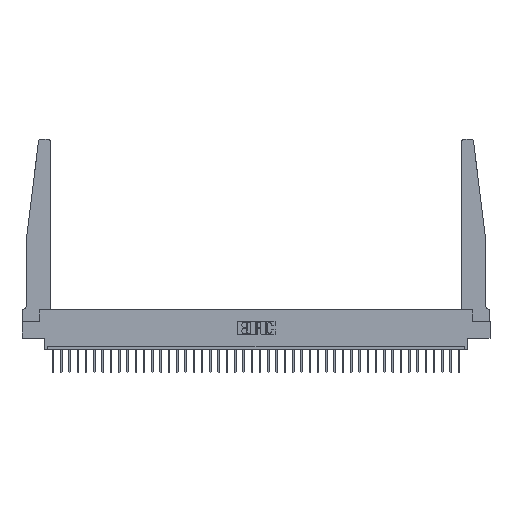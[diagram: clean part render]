
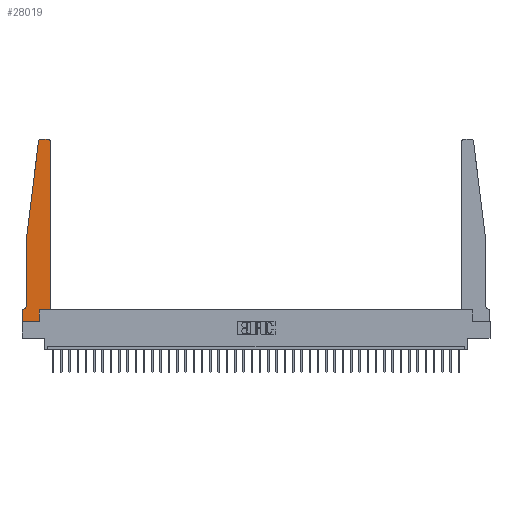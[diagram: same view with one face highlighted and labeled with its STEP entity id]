
A CAD part, top view. The second image highlights one B-rep face of the part: STEP entity #28019.
In plain terms, the highlighted planar face has unit normal (0, 0, 1).
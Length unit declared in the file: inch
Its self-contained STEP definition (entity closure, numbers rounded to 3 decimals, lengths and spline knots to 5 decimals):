
#20 = CARTESIAN_POINT ( 'NONE',  ( 0.015, 0.2375, 0.37 ) ) ;
#563 = EDGE_CURVE ( 'NONE', #23063, #26368, #12569, .T. ) ;
#759 = CARTESIAN_POINT ( 'NONE',  ( 0.425, 0.18, 0.37 ) ) ;
#1128 = CARTESIAN_POINT ( 'NONE',  ( 0.425, 0.18, 0.37 ) ) ;
#1608 = CARTESIAN_POINT ( 'NONE',  ( 0.27653, 2.75, 0.37 ) ) ;
#1908 = LINE ( 'NONE', #4752, #3037 ) ;
#2266 = EDGE_CURVE ( 'NONE', #28816, #15659, #31249, .T. ) ;
#2696 = DIRECTION ( 'NONE',  ( 0., 0., -1. ) ) ;
#2942 = ORIENTED_EDGE ( 'NONE', *, *, #29391, .T. ) ;
#2980 = EDGE_CURVE ( 'NONE', #21040, #24756, #8687, .T. ) ;
#3037 = VECTOR ( 'NONE', #24036, 39.37008 ) ;
#3218 = VERTEX_POINT ( 'NONE', #23481 ) ;
#4462 = LINE ( 'NONE', #7508, #11585 ) ;
#4684 = VERTEX_POINT ( 'NONE', #16471 ) ;
#4752 = CARTESIAN_POINT ( 'NONE',  ( 0.25, 2.75, 0.37 ) ) ;
#4827 = VECTOR ( 'NONE', #22648, 39.37008 ) ;
#4840 = ORIENTED_EDGE ( 'NONE', *, *, #563, .T. ) ;
#4937 = DIRECTION ( 'NONE',  ( 1., 0., 0. ) ) ;
#5009 = ORIENTED_EDGE ( 'NONE', *, *, #22281, .T. ) ;
#5348 = VECTOR ( 'NONE', #34368, 39.37008 ) ;
#5630 = DIRECTION ( 'NONE',  ( 0., 0., 1. ) ) ;
#5675 = EDGE_CURVE ( 'NONE', #25579, #21040, #12344, .T. ) ;
#5929 = ORIENTED_EDGE ( 'NONE', *, *, #35224, .T. ) ;
#6395 = VECTOR ( 'NONE', #9640, 39.37008 ) ;
#6528 = ORIENTED_EDGE ( 'NONE', *, *, #2980, .T. ) ;
#6663 = CARTESIAN_POINT ( 'NONE',  ( 0.425, 0.18, 0.37 ) ) ;
#6870 = LINE ( 'NONE', #7040, #10419 ) ;
#6914 = VECTOR ( 'NONE', #19304, 39.37008 ) ;
#7040 = CARTESIAN_POINT ( 'NONE',  ( 0., 0., 0.37 ) ) ;
#7508 = CARTESIAN_POINT ( 'NONE',  ( 0., 0., 0.37 ) ) ;
#8687 = CIRCLE ( 'NONE', #12109, 0.03 ) ;
#9262 = CARTESIAN_POINT ( 'NONE',  ( 0.065, 1.25, 0.37 ) ) ;
#9301 = AXIS2_PLACEMENT_3D ( 'NONE', #21191, #19019, #4937 ) ;
#9640 = DIRECTION ( 'NONE',  ( -1., 0., 0. ) ) ;
#9796 = VERTEX_POINT ( 'NONE', #22073 ) ;
#10419 = VECTOR ( 'NONE', #31155, 39.37008 ) ;
#11344 = CARTESIAN_POINT ( 'NONE',  ( 0.395, 2.72, 0.37 ) ) ;
#11585 = VECTOR ( 'NONE', #26605, 39.37008 ) ;
#11973 = EDGE_CURVE ( 'NONE', #3218, #25579, #14313, .T. ) ;
#12001 = DIRECTION ( 'NONE',  ( 0., 1., 0. ) ) ;
#12109 = AXIS2_PLACEMENT_3D ( 'NONE', #11344, #5630, #19182 ) ;
#12344 = LINE ( 'NONE', #1128, #35107 ) ;
#12569 = LINE ( 'NONE', #23465, #5348 ) ;
#14114 = CIRCLE ( 'NONE', #20486, 0.03 ) ;
#14313 = LINE ( 'NONE', #759, #6914 ) ;
#14477 = EDGE_LOOP ( 'NONE', ( #32243, #5009, #15968, #4840, #5929, #16806, #2942, #17215, #19859, #19806, #26838, #6528 ) ) ;
#14504 = VECTOR ( 'NONE', #22470, 39.37008 ) ;
#14520 = CIRCLE ( 'NONE', #19070, 0.05 ) ;
#14826 = CARTESIAN_POINT ( 'NONE',  ( 0.425, 2.72, 0.37 ) ) ;
#15659 = VERTEX_POINT ( 'NONE', #32582 ) ;
#15968 = ORIENTED_EDGE ( 'NONE', *, *, #33214, .T. ) ;
#16471 = CARTESIAN_POINT ( 'NONE',  ( 0.24675, 2.72367, 0.37 ) ) ;
#16806 = ORIENTED_EDGE ( 'NONE', *, *, #2266, .T. ) ;
#16820 = EDGE_CURVE ( 'NONE', #24756, #31630, #1908, .T. ) ;
#17215 = ORIENTED_EDGE ( 'NONE', *, *, #28623, .T. ) ;
#18679 = PLANE ( 'NONE',  #9301 ) ;
#18930 = CARTESIAN_POINT ( 'NONE',  ( 0.27653, 2.72, 0.37 ) ) ;
#19019 = DIRECTION ( 'NONE',  ( 0., 0., 1. ) ) ;
#19070 = AXIS2_PLACEMENT_3D ( 'NONE', #20, #2696, #21448 ) ;
#19182 = DIRECTION ( 'NONE',  ( 1., 0., 0. ) ) ;
#19304 = DIRECTION ( 'NONE',  ( 1., 0., 0. ) ) ;
#19806 = ORIENTED_EDGE ( 'NONE', *, *, #11973, .T. ) ;
#19859 = ORIENTED_EDGE ( 'NONE', *, *, #33170, .T. ) ;
#19967 = LINE ( 'NONE', #9262, #4827 ) ;
#20138 = LINE ( 'NONE', #28366, #14504 ) ;
#20486 = AXIS2_PLACEMENT_3D ( 'NONE', #18930, #24476, #33044 ) ;
#21040 = VERTEX_POINT ( 'NONE', #14826 ) ;
#21191 = CARTESIAN_POINT ( 'NONE',  ( 0., 0.1875, 0.37 ) ) ;
#21448 = DIRECTION ( 'NONE',  ( -1., 0., 0. ) ) ;
#22073 = CARTESIAN_POINT ( 'NONE',  ( 0., 0., 0.37 ) ) ;
#22281 = EDGE_CURVE ( 'NONE', #31630, #4684, #14114, .T. ) ;
#22470 = DIRECTION ( 'NONE',  ( 0., 1., 0. ) ) ;
#22648 = DIRECTION ( 'NONE',  ( -0.122, -0.992, 0. ) ) ;
#22893 = VERTEX_POINT ( 'NONE', #26209 ) ;
#23063 = VERTEX_POINT ( 'NONE', #24390 ) ;
#23465 = CARTESIAN_POINT ( 'NONE',  ( 0.065, 1.25, 0.37 ) ) ;
#23481 = CARTESIAN_POINT ( 'NONE',  ( 0.2605, 0.18, 0.37 ) ) ;
#24020 = CARTESIAN_POINT ( 'NONE',  ( 0.395, 2.75, 0.37 ) ) ;
#24036 = DIRECTION ( 'NONE',  ( -1., 0., 0. ) ) ;
#24049 = FACE_OUTER_BOUND ( 'NONE', #14477, .T. ) ;
#24390 = CARTESIAN_POINT ( 'NONE',  ( 0.065, 1.25, 0.37 ) ) ;
#24476 = DIRECTION ( 'NONE',  ( 0., 0., 1. ) ) ;
#24756 = VERTEX_POINT ( 'NONE', #24020 ) ;
#25579 = VERTEX_POINT ( 'NONE', #6663 ) ;
#25887 = CARTESIAN_POINT ( 'NONE',  ( 0.065, 0.1875, 0.37 ) ) ;
#26209 = CARTESIAN_POINT ( 'NONE',  ( 0.2605, 0., 0.37 ) ) ;
#26368 = VERTEX_POINT ( 'NONE', #33670 ) ;
#26605 = DIRECTION ( 'NONE',  ( 1., 0., 0. ) ) ;
#26838 = ORIENTED_EDGE ( 'NONE', *, *, #5675, .T. ) ;
#28019 = ADVANCED_FACE ( 'NONE', ( #24049 ), #18679, .T. ) ;
#28366 = CARTESIAN_POINT ( 'NONE',  ( 0.2605, 0.18, 0.37 ) ) ;
#28623 = EDGE_CURVE ( 'NONE', #9796, #22893, #4462, .T. ) ;
#28816 = VERTEX_POINT ( 'NONE', #33730 ) ;
#29391 = EDGE_CURVE ( 'NONE', #15659, #9796, #6870, .T. ) ;
#31155 = DIRECTION ( 'NONE',  ( 0., -1., 0. ) ) ;
#31249 = LINE ( 'NONE', #25887, #6395 ) ;
#31630 = VERTEX_POINT ( 'NONE', #1608 ) ;
#32243 = ORIENTED_EDGE ( 'NONE', *, *, #16820, .T. ) ;
#32582 = CARTESIAN_POINT ( 'NONE',  ( 0., 0.1875, 0.37 ) ) ;
#33044 = DIRECTION ( 'NONE',  ( 1., 0., 0. ) ) ;
#33170 = EDGE_CURVE ( 'NONE', #22893, #3218, #20138, .T. ) ;
#33214 = EDGE_CURVE ( 'NONE', #4684, #23063, #19967, .T. ) ;
#33670 = CARTESIAN_POINT ( 'NONE',  ( 0.065, 0.2375, 0.37 ) ) ;
#33730 = CARTESIAN_POINT ( 'NONE',  ( 0.015, 0.1875, 0.37 ) ) ;
#34368 = DIRECTION ( 'NONE',  ( 0., -1., 0. ) ) ;
#35107 = VECTOR ( 'NONE', #12001, 39.37008 ) ;
#35224 = EDGE_CURVE ( 'NONE', #26368, #28816, #14520, .T. ) ;
